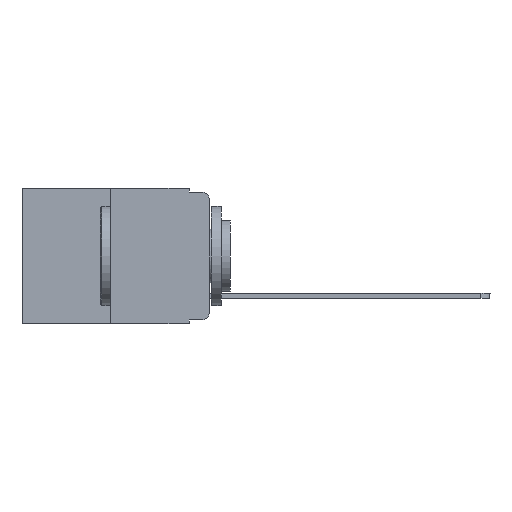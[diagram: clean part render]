
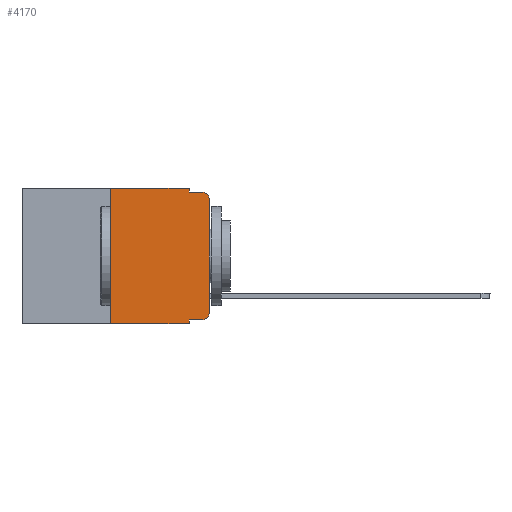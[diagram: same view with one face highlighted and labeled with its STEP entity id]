
A CAD part, left-side view. The second image highlights one B-rep face of the part: STEP entity #4170.
In plain terms, the highlighted planar face has unit normal (-1, 0, 0).
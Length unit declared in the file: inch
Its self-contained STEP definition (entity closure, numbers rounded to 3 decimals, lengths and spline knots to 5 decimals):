
#23 = CARTESIAN_POINT ( 'NONE',  ( 0., 0.25, 0. ) ) ;
#62 = CARTESIAN_POINT ( 'NONE',  ( 0., 0.25, 0. ) ) ;
#77 = CARTESIAN_POINT ( 'NONE',  ( 0., 0.051, -0.01 ) ) ;
#325 = VERTEX_POINT ( 'NONE', #8243 ) ;
#447 = LINE ( 'NONE', #7673, #1280 ) ;
#518 = EDGE_CURVE ( 'NONE', #4261, #614, #4244, .T. ) ;
#614 = VERTEX_POINT ( 'NONE', #62 ) ;
#882 = LINE ( 'NONE', #7819, #1561 ) ;
#1099 = CARTESIAN_POINT ( 'NONE',  ( 0., 0.473, 0. ) ) ;
#1200 = LINE ( 'NONE', #1099, #2979 ) ;
#1280 = VECTOR ( 'NONE', #8482, 39.37008 ) ;
#1401 = FACE_OUTER_BOUND ( 'NONE', #5824, .T. ) ;
#1507 = EDGE_CURVE ( 'NONE', #614, #325, #1200, .T. ) ;
#1561 = VECTOR ( 'NONE', #3190, 39.37008 ) ;
#1673 = ORIENTED_EDGE ( 'NONE', *, *, #4301, .T. ) ;
#2073 = CARTESIAN_POINT ( 'NONE',  ( 0., 0., -0.03 ) ) ;
#2079 = ORIENTED_EDGE ( 'NONE', *, *, #7531, .T. ) ;
#2519 = EDGE_CURVE ( 'NONE', #6381, #4124, #882, .T. ) ;
#2559 = VERTEX_POINT ( 'NONE', #2073 ) ;
#2625 = CARTESIAN_POINT ( 'NONE',  ( 0., 0.25, -0.343 ) ) ;
#2979 = VECTOR ( 'NONE', #6463, 39.37008 ) ;
#3114 = DIRECTION ( 'NONE',  ( 0., 0., -1. ) ) ;
#3190 = DIRECTION ( 'NONE',  ( 0., -1., 0. ) ) ;
#3254 = AXIS2_PLACEMENT_3D ( 'NONE', #5131, #8592, #3407 ) ;
#3407 = DIRECTION ( 'NONE',  ( 0., 0., -1. ) ) ;
#3437 = EDGE_CURVE ( 'NONE', #6381, #11159, #447, .T. ) ;
#3527 = DIRECTION ( 'NONE',  ( 0., -1., 0. ) ) ;
#3758 = EDGE_CURVE ( 'NONE', #325, #7991, #5005, .T. ) ;
#3762 = ORIENTED_EDGE ( 'NONE', *, *, #4042, .T. ) ;
#3822 = CARTESIAN_POINT ( 'NONE',  ( 0., 0.051, -0.01 ) ) ;
#4042 = EDGE_CURVE ( 'NONE', #4124, #7430, #9507, .T. ) ;
#4106 = DIRECTION ( 'NONE',  ( -1., 0., 0. ) ) ;
#4124 = VERTEX_POINT ( 'NONE', #8555 ) ;
#4170 = ADVANCED_FACE ( 'NONE', ( #1401 ), #7747, .F. ) ;
#4244 = LINE ( 'NONE', #23, #8486 ) ;
#4261 = VERTEX_POINT ( 'NONE', #2625 ) ;
#4299 = LINE ( 'NONE', #5290, #8135 ) ;
#4301 = EDGE_CURVE ( 'NONE', #4261, #11159, #4299, .T. ) ;
#5005 = LINE ( 'NONE', #6625, #11136 ) ;
#5131 = CARTESIAN_POINT ( 'NONE',  ( 0., 0.473, 0. ) ) ;
#5290 = CARTESIAN_POINT ( 'NONE',  ( 0., 0.473, -0.343 ) ) ;
#5350 = VECTOR ( 'NONE', #10723, 39.37008 ) ;
#5385 = CARTESIAN_POINT ( 'NONE',  ( 0., 0.051, -0.343 ) ) ;
#5434 = AXIS2_PLACEMENT_3D ( 'NONE', #8682, #6105, #6950 ) ;
#5640 = CARTESIAN_POINT ( 'NONE',  ( 0., 0., -0.313 ) ) ;
#5824 = EDGE_LOOP ( 'NONE', ( #7439, #2079, #8450, #6451, #7903, #11041, #1673, #6171, #10951, #3762 ) ) ;
#5903 = LINE ( 'NONE', #77, #5350 ) ;
#5909 = VERTEX_POINT ( 'NONE', #9499 ) ;
#6105 = DIRECTION ( 'NONE',  ( -1., 0., 0. ) ) ;
#6171 = ORIENTED_EDGE ( 'NONE', *, *, #3437, .F. ) ;
#6182 = DIRECTION ( 'NONE',  ( 0., 0., 1. ) ) ;
#6381 = VERTEX_POINT ( 'NONE', #11233 ) ;
#6451 = ORIENTED_EDGE ( 'NONE', *, *, #3758, .F. ) ;
#6462 = EDGE_CURVE ( 'NONE', #7430, #2559, #11354, .T. ) ;
#6463 = DIRECTION ( 'NONE',  ( 0., -1., 0. ) ) ;
#6625 = CARTESIAN_POINT ( 'NONE',  ( 0., 0.051, 0. ) ) ;
#6675 = DIRECTION ( 'NONE',  ( 0., 0., -1. ) ) ;
#6950 = DIRECTION ( 'NONE',  ( 0., 0., -1. ) ) ;
#7200 = EDGE_CURVE ( 'NONE', #7991, #5909, #5903, .T. ) ;
#7430 = VERTEX_POINT ( 'NONE', #5640 ) ;
#7439 = ORIENTED_EDGE ( 'NONE', *, *, #6462, .T. ) ;
#7531 = EDGE_CURVE ( 'NONE', #2559, #5909, #7605, .T. ) ;
#7605 = CIRCLE ( 'NONE', #11144, 0.02 ) ;
#7673 = CARTESIAN_POINT ( 'NONE',  ( 0., 0.051, 0. ) ) ;
#7696 = CARTESIAN_POINT ( 'NONE',  ( 0., 0.02, -0.03 ) ) ;
#7723 = CARTESIAN_POINT ( 'NONE',  ( 0., 0., 0. ) ) ;
#7747 = PLANE ( 'NONE',  #3254 ) ;
#7819 = CARTESIAN_POINT ( 'NONE',  ( 0., 0.051, -0.333 ) ) ;
#7903 = ORIENTED_EDGE ( 'NONE', *, *, #1507, .F. ) ;
#7991 = VERTEX_POINT ( 'NONE', #3822 ) ;
#8135 = VECTOR ( 'NONE', #3527, 39.37008 ) ;
#8243 = CARTESIAN_POINT ( 'NONE',  ( 0., 0.051, 0. ) ) ;
#8450 = ORIENTED_EDGE ( 'NONE', *, *, #7200, .F. ) ;
#8482 = DIRECTION ( 'NONE',  ( 0., 0., -1. ) ) ;
#8486 = VECTOR ( 'NONE', #6182, 39.37008 ) ;
#8555 = CARTESIAN_POINT ( 'NONE',  ( 0., 0.02, -0.333 ) ) ;
#8592 = DIRECTION ( 'NONE',  ( 1., 0., 0. ) ) ;
#8682 = CARTESIAN_POINT ( 'NONE',  ( 0., 0.02, -0.313 ) ) ;
#9447 = DIRECTION ( 'NONE',  ( 0., 0., 1. ) ) ;
#9499 = CARTESIAN_POINT ( 'NONE',  ( 0., 0.02, -0.01 ) ) ;
#9507 = CIRCLE ( 'NONE', #5434, 0.02 ) ;
#10519 = VECTOR ( 'NONE', #9447, 39.37008 ) ;
#10723 = DIRECTION ( 'NONE',  ( 0., -1., 0. ) ) ;
#10951 = ORIENTED_EDGE ( 'NONE', *, *, #2519, .T. ) ;
#11041 = ORIENTED_EDGE ( 'NONE', *, *, #518, .F. ) ;
#11136 = VECTOR ( 'NONE', #3114, 39.37008 ) ;
#11144 = AXIS2_PLACEMENT_3D ( 'NONE', #7696, #4106, #6675 ) ;
#11159 = VERTEX_POINT ( 'NONE', #5385 ) ;
#11233 = CARTESIAN_POINT ( 'NONE',  ( 0., 0.051, -0.333 ) ) ;
#11354 = LINE ( 'NONE', #7723, #10519 ) ;
